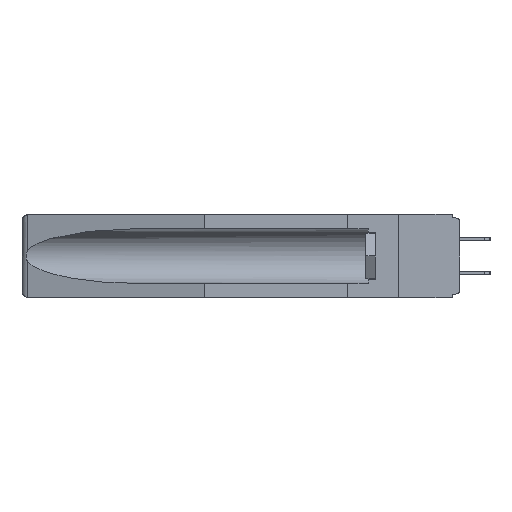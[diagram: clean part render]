
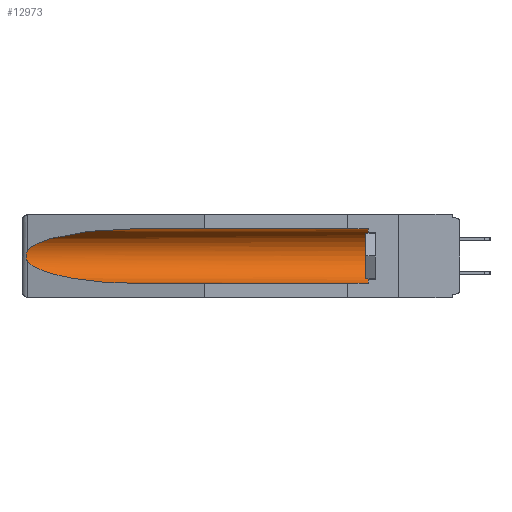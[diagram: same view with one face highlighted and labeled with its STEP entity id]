
A CAD part, left-side view. The second image highlights one B-rep face of the part: STEP entity #12973.
In plain terms, the highlighted cylindrical face has radius 2.857 mm (diameter 5.715 mm), a partial arc.
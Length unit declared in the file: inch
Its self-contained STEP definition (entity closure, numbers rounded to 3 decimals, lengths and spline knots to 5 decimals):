
#1403 = CARTESIAN_POINT ( 'NONE',  ( 0.26537, 1.52718, -0.14972 ) ) ;
#1691 = CARTESIAN_POINT ( 'NONE',  ( 0.26537, 1.52718, -0.14972 ) ) ;
#1817 = CYLINDRICAL_SURFACE ( 'NONE', #8187, 0.1125 ) ;
#1823 = DIRECTION ( 'NONE',  ( 0., 0., 1. ) ) ;
#1919 = VERTEX_POINT ( 'NONE', #1691 ) ;
#2140 = CARTESIAN_POINT ( 'NONE',  ( 0.2673, 1.53269, -0.17917 ) ) ;
#2868 = EDGE_CURVE ( 'NONE', #6566, #9536, #11959, .T. ) ;
#3239 = CARTESIAN_POINT ( 'NONE',  ( 0.21114, 1.30732, -0.059 ) ) ;
#3766 = CARTESIAN_POINT ( 'NONE',  ( 0.155, -0.30754, -0.1715 ) ) ;
#4985 = CARTESIAN_POINT ( 'NONE',  ( 0.21114, 1.30732, -0.284 ) ) ;
#5330 = LINE ( 'NONE', #15982, #22704 ) ;
#5363 = ORIENTED_EDGE ( 'NONE', *, *, #2868, .T. ) ;
#5636 = CARTESIAN_POINT ( 'NONE',  ( 0.2675, 1.53308, -0.16763 ) ) ;
#6106 = CARTESIAN_POINT ( 'NONE',  ( 0.155, 0.126, -0.284 ) ) ;
#6456 = ORIENTED_EDGE ( 'NONE', *, *, #6929, .F. ) ;
#6566 = VERTEX_POINT ( 'NONE', #14517 ) ;
#6929 = EDGE_CURVE ( 'NONE', #10450, #9536, #5330, .T. ) ;
#7245 = CARTESIAN_POINT ( 'NONE',  ( 0.155, -0.30754, -0.059 ) ) ;
#7427 = EDGE_LOOP ( 'NONE', ( #13121, #17396, #5363, #6456, #8850, #19115 ) ) ;
#7645 = FACE_OUTER_BOUND ( 'NONE', #7427, .T. ) ;
#7812 = CARTESIAN_POINT ( 'NONE',  ( 0.155, 0.126, -0.059 ) ) ;
#7879 = VERTEX_POINT ( 'NONE', #7812 ) ;
#8187 = AXIS2_PLACEMENT_3D ( 'NONE', #3766, #12544, #14155 ) ;
#8850 = ORIENTED_EDGE ( 'NONE', *, *, #22796, .T. ) ;
#9303 =( BOUNDED_CURVE ( )  B_SPLINE_CURVE ( 3, ( #10173, #3239, #18863, #1403 ),
 .UNSPECIFIED., .F., .F. ) 
 B_SPLINE_CURVE_WITH_KNOTS ( ( 4, 4 ),
 ( 4.71239, 6.08839 ),
 .UNSPECIFIED. ) 
 CURVE ( )  GEOMETRIC_REPRESENTATION_ITEM ( )  RATIONAL_B_SPLINE_CURVE ( ( 1., 0.848, 0.848, 1. ) ) 
 REPRESENTATION_ITEM ( '' )  );
#9536 = VERTEX_POINT ( 'NONE', #14065 ) ;
#9655 = CIRCLE ( 'NONE', #12793, 0.1125 ) ;
#10173 = CARTESIAN_POINT ( 'NONE',  ( 0.155, 1.07973, -0.059 ) ) ;
#10450 = VERTEX_POINT ( 'NONE', #6106 ) ;
#10749 = DIRECTION ( 'NONE',  ( 0., -1., 0. ) ) ;
#10836 = CARTESIAN_POINT ( 'NONE',  ( 0.26597, 1.52961, -0.15275 ) ) ;
#10919 = CARTESIAN_POINT ( 'NONE',  ( 0.2675, 1.53308, -0.17534 ) ) ;
#11843 = VECTOR ( 'NONE', #19387, 39.37008 ) ;
#11959 =( BOUNDED_CURVE ( )  B_SPLINE_CURVE ( 3, ( #22545, #13813, #4985, #11965 ),
 .UNSPECIFIED., .F., .F. ) 
 B_SPLINE_CURVE_WITH_KNOTS ( ( 4, 4 ),
 ( 0.1948, 1.5708 ),
 .UNSPECIFIED. ) 
 CURVE ( )  GEOMETRIC_REPRESENTATION_ITEM ( )  RATIONAL_B_SPLINE_CURVE ( ( 1., 0.848, 0.848, 1. ) ) 
 REPRESENTATION_ITEM ( '' )  );
#11965 = CARTESIAN_POINT ( 'NONE',  ( 0.155, 1.07973, -0.284 ) ) ;
#12444 = CARTESIAN_POINT ( 'NONE',  ( 0.155, 0.126, -0.1715 ) ) ;
#12544 = DIRECTION ( 'NONE',  ( 0., 1., 0. ) ) ;
#12561 = DIRECTION ( 'NONE',  ( 0., 1., 0. ) ) ;
#12619 = CARTESIAN_POINT ( 'NONE',  ( 0.26654, 1.53092, -0.15636 ) ) ;
#12793 = AXIS2_PLACEMENT_3D ( 'NONE', #12444, #10749, #1823 ) ;
#12973 = ADVANCED_FACE ( 'NONE', ( #7645 ), #1817, .F. ) ;
#13121 = ORIENTED_EDGE ( 'NONE', *, *, #15210, .T. ) ;
#13813 = CARTESIAN_POINT ( 'NONE',  ( 0.25451, 1.48313, -0.24835 ) ) ;
#14065 = CARTESIAN_POINT ( 'NONE',  ( 0.155, 1.07973, -0.284 ) ) ;
#14155 = DIRECTION ( 'NONE',  ( 0., 0., 1. ) ) ;
#14517 = CARTESIAN_POINT ( 'NONE',  ( 0.26537, 1.52718, -0.19328 ) ) ;
#14583 = LINE ( 'NONE', #7245, #11843 ) ;
#15210 = EDGE_CURVE ( 'NONE', #21914, #1919, #9303, .T. ) ;
#15310 = B_SPLINE_CURVE_WITH_KNOTS ( 'NONE', 3,
 ( #16112, #10836, #12619, #21630, #5636, #10919, #2140, #17983, #20008, #20325 ),
 .UNSPECIFIED., .F., .F.,
 ( 4, 2, 2, 2, 4 ),
 ( 0., 0.00029, 0.00058, 0.00087, 0.00117 ),
 .UNSPECIFIED. ) ;
#15982 = CARTESIAN_POINT ( 'NONE',  ( 0.155, -0.30754, -0.284 ) ) ;
#16112 = CARTESIAN_POINT ( 'NONE',  ( 0.26537, 1.52718, -0.14972 ) ) ;
#16902 = CARTESIAN_POINT ( 'NONE',  ( 0.155, 1.07973, -0.059 ) ) ;
#17396 = ORIENTED_EDGE ( 'NONE', *, *, #20610, .T. ) ;
#17983 = CARTESIAN_POINT ( 'NONE',  ( 0.26655, 1.53094, -0.18657 ) ) ;
#18863 = CARTESIAN_POINT ( 'NONE',  ( 0.25451, 1.48313, -0.09465 ) ) ;
#19115 = ORIENTED_EDGE ( 'NONE', *, *, #22777, .T. ) ;
#19387 = DIRECTION ( 'NONE',  ( 0., 1., 0. ) ) ;
#20008 = CARTESIAN_POINT ( 'NONE',  ( 0.26597, 1.5296, -0.19026 ) ) ;
#20325 = CARTESIAN_POINT ( 'NONE',  ( 0.26537, 1.52718, -0.19328 ) ) ;
#20610 = EDGE_CURVE ( 'NONE', #1919, #6566, #15310, .T. ) ;
#21630 = CARTESIAN_POINT ( 'NONE',  ( 0.2673, 1.5327, -0.16383 ) ) ;
#21914 = VERTEX_POINT ( 'NONE', #16902 ) ;
#22545 = CARTESIAN_POINT ( 'NONE',  ( 0.26537, 1.52718, -0.19328 ) ) ;
#22704 = VECTOR ( 'NONE', #12561, 39.37008 ) ;
#22777 = EDGE_CURVE ( 'NONE', #7879, #21914, #14583, .T. ) ;
#22796 = EDGE_CURVE ( 'NONE', #10450, #7879, #9655, .T. ) ;
